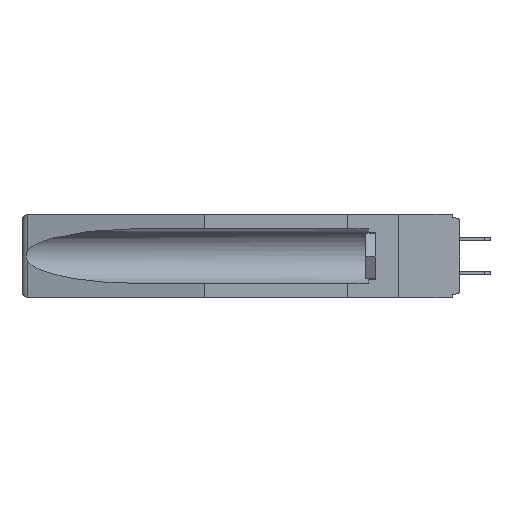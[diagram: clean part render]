
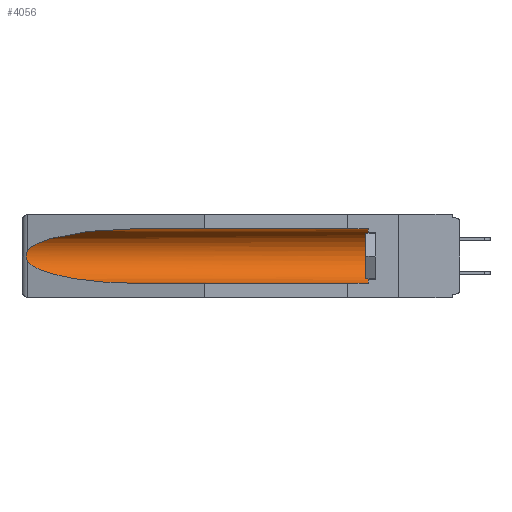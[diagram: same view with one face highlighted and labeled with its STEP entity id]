
A CAD part, left-side view. The second image highlights one B-rep face of the part: STEP entity #4056.
In plain terms, the highlighted cylindrical face has radius 2.857 mm (diameter 5.715 mm), a partial arc.
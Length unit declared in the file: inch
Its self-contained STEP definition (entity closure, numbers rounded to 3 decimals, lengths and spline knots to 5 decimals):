
#350 = CARTESIAN_POINT ( 'NONE',  ( 0.26597, 1.52961, -0.15275 ) ) ;
#648 = CARTESIAN_POINT ( 'NONE',  ( 0.155, 1.07973, -0.059 ) ) ;
#954 = CARTESIAN_POINT ( 'NONE',  ( 0.26537, 1.52718, -0.14972 ) ) ;
#1286 = ORIENTED_EDGE ( 'NONE', *, *, #19794, .T. ) ;
#2410 = VERTEX_POINT ( 'NONE', #16157 ) ;
#2485 = CARTESIAN_POINT ( 'NONE',  ( 0.26537, 1.52718, -0.19328 ) ) ;
#2504 = EDGE_CURVE ( 'NONE', #2410, #11691, #18522, .T. ) ;
#2835 = CARTESIAN_POINT ( 'NONE',  ( 0.155, 1.07973, -0.284 ) ) ;
#3304 = DIRECTION ( 'NONE',  ( 0., 0., 1. ) ) ;
#3311 = CARTESIAN_POINT ( 'NONE',  ( 0.155, -0.30754, -0.059 ) ) ;
#3945 = DIRECTION ( 'NONE',  ( 0., 1., 0. ) ) ;
#4056 = ADVANCED_FACE ( 'NONE', ( #25850 ), #24885, .F. ) ;
#4941 = ORIENTED_EDGE ( 'NONE', *, *, #12795, .T. ) ;
#4953 = VECTOR ( 'NONE', #3945, 39.37008 ) ;
#5177 = CARTESIAN_POINT ( 'NONE',  ( 0.2675, 1.53308, -0.16763 ) ) ;
#6163 = VECTOR ( 'NONE', #21352, 39.37008 ) ;
#6509 = EDGE_CURVE ( 'NONE', #11497, #2410, #26012, .T. ) ;
#6527 = ORIENTED_EDGE ( 'NONE', *, *, #21088, .F. ) ;
#7150 = AXIS2_PLACEMENT_3D ( 'NONE', #7703, #20280, #7977 ) ;
#7703 = CARTESIAN_POINT ( 'NONE',  ( 0.155, -0.30754, -0.1715 ) ) ;
#7977 = DIRECTION ( 'NONE',  ( 0., 0., 1. ) ) ;
#8788 = CARTESIAN_POINT ( 'NONE',  ( 0.155, 1.07973, -0.284 ) ) ;
#9284 = CARTESIAN_POINT ( 'NONE',  ( 0.155, 0.126, -0.1715 ) ) ;
#9364 = CARTESIAN_POINT ( 'NONE',  ( 0.26597, 1.5296, -0.19026 ) ) ;
#9627 =( BOUNDED_CURVE ( )  B_SPLINE_CURVE ( 3, ( #24701, #24539, #16166, #12013 ),
 .UNSPECIFIED., .F., .F. ) 
 B_SPLINE_CURVE_WITH_KNOTS ( ( 4, 4 ),
 ( 4.71239, 6.08839 ),
 .UNSPECIFIED. ) 
 CURVE ( )  GEOMETRIC_REPRESENTATION_ITEM ( )  RATIONAL_B_SPLINE_CURVE ( ( 1., 0.848, 0.848, 1. ) ) 
 REPRESENTATION_ITEM ( '' )  );
#11497 = VERTEX_POINT ( 'NONE', #24354 ) ;
#11691 = VERTEX_POINT ( 'NONE', #648 ) ;
#12013 = CARTESIAN_POINT ( 'NONE',  ( 0.26537, 1.52718, -0.14972 ) ) ;
#12080 = VERTEX_POINT ( 'NONE', #20785 ) ;
#12095 = CARTESIAN_POINT ( 'NONE',  ( 0.26537, 1.52718, -0.19328 ) ) ;
#12795 = EDGE_CURVE ( 'NONE', #11691, #12080, #9627, .T. ) ;
#12938 = CARTESIAN_POINT ( 'NONE',  ( 0.21114, 1.30732, -0.284 ) ) ;
#13583 = DIRECTION ( 'NONE',  ( 0., -1., 0. ) ) ;
#15247 = CARTESIAN_POINT ( 'NONE',  ( 0.155, -0.30754, -0.284 ) ) ;
#15408 = VERTEX_POINT ( 'NONE', #2835 ) ;
#16157 = CARTESIAN_POINT ( 'NONE',  ( 0.155, 0.126, -0.059 ) ) ;
#16166 = CARTESIAN_POINT ( 'NONE',  ( 0.25451, 1.48313, -0.09465 ) ) ;
#16813 = VERTEX_POINT ( 'NONE', #12095 ) ;
#17524 = CARTESIAN_POINT ( 'NONE',  ( 0.26654, 1.53092, -0.15636 ) ) ;
#18522 = LINE ( 'NONE', #3311, #4953 ) ;
#18923 = ORIENTED_EDGE ( 'NONE', *, *, #6509, .T. ) ;
#19039 = CARTESIAN_POINT ( 'NONE',  ( 0.2673, 1.5327, -0.16383 ) ) ;
#19794 = EDGE_CURVE ( 'NONE', #16813, #15408, #25618, .T. ) ;
#20280 = DIRECTION ( 'NONE',  ( 0., 1., 0. ) ) ;
#20785 = CARTESIAN_POINT ( 'NONE',  ( 0.26537, 1.52718, -0.14972 ) ) ;
#21088 = EDGE_CURVE ( 'NONE', #11497, #15408, #22277, .T. ) ;
#21119 = ORIENTED_EDGE ( 'NONE', *, *, #22247, .T. ) ;
#21352 = DIRECTION ( 'NONE',  ( 0., 1., 0. ) ) ;
#21659 = CARTESIAN_POINT ( 'NONE',  ( 0.2673, 1.53269, -0.17917 ) ) ;
#22247 = EDGE_CURVE ( 'NONE', #12080, #16813, #22300, .T. ) ;
#22277 = LINE ( 'NONE', #15247, #6163 ) ;
#22300 = B_SPLINE_CURVE_WITH_KNOTS ( 'NONE', 3,
 ( #954, #350, #17524, #19039, #5177, #22986, #21659, #23647, #9364, #2485 ),
 .UNSPECIFIED., .F., .F.,
 ( 4, 2, 2, 2, 4 ),
 ( 0., 0.00029, 0.00058, 0.00087, 0.00117 ),
 .UNSPECIFIED. ) ;
#22986 = CARTESIAN_POINT ( 'NONE',  ( 0.2675, 1.53308, -0.17534 ) ) ;
#23164 = CARTESIAN_POINT ( 'NONE',  ( 0.26537, 1.52718, -0.19328 ) ) ;
#23255 = CARTESIAN_POINT ( 'NONE',  ( 0.25451, 1.48313, -0.24835 ) ) ;
#23647 = CARTESIAN_POINT ( 'NONE',  ( 0.26655, 1.53094, -0.18657 ) ) ;
#23826 = ORIENTED_EDGE ( 'NONE', *, *, #2504, .T. ) ;
#24354 = CARTESIAN_POINT ( 'NONE',  ( 0.155, 0.126, -0.284 ) ) ;
#24539 = CARTESIAN_POINT ( 'NONE',  ( 0.21114, 1.30732, -0.059 ) ) ;
#24701 = CARTESIAN_POINT ( 'NONE',  ( 0.155, 1.07973, -0.059 ) ) ;
#24885 = CYLINDRICAL_SURFACE ( 'NONE', #7150, 0.1125 ) ;
#25618 =( BOUNDED_CURVE ( )  B_SPLINE_CURVE ( 3, ( #23164, #23255, #12938, #8788 ),
 .UNSPECIFIED., .F., .T. ) 
 B_SPLINE_CURVE_WITH_KNOTS ( ( 4, 4 ),
 ( 0.1948, 1.5708 ),
 .UNSPECIFIED. ) 
 CURVE ( )  GEOMETRIC_REPRESENTATION_ITEM ( )  RATIONAL_B_SPLINE_CURVE ( ( 1., 0.848, 0.848, 1. ) ) 
 REPRESENTATION_ITEM ( '' )  );
#25816 = AXIS2_PLACEMENT_3D ( 'NONE', #9284, #13583, #3304 ) ;
#25850 = FACE_OUTER_BOUND ( 'NONE', #26169, .T. ) ;
#26012 = CIRCLE ( 'NONE', #25816, 0.1125 ) ;
#26169 = EDGE_LOOP ( 'NONE', ( #4941, #21119, #1286, #6527, #18923, #23826 ) ) ;
